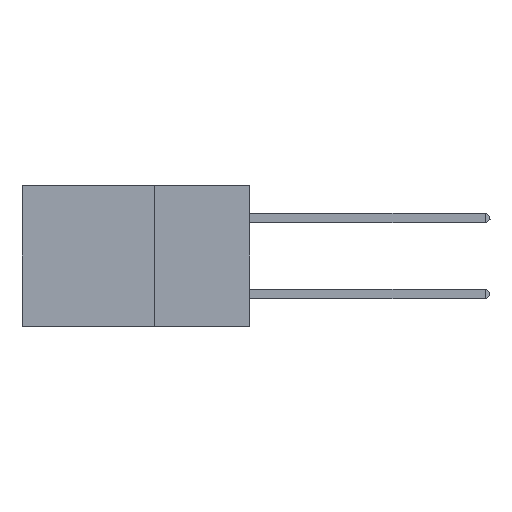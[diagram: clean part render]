
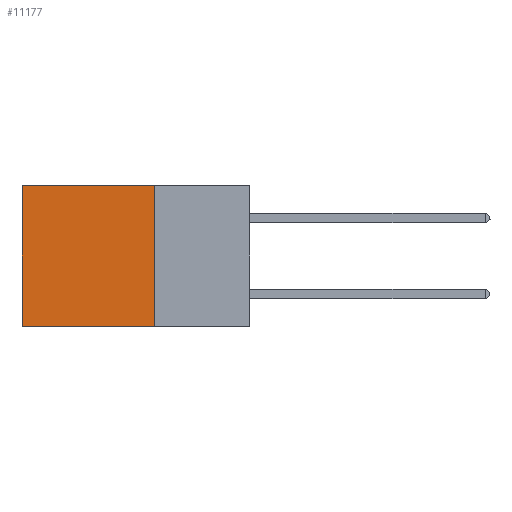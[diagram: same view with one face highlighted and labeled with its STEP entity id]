
A CAD part, left-side view. The second image highlights one B-rep face of the part: STEP entity #11177.
In plain terms, the highlighted planar face has unit normal (-1, 0, 0).
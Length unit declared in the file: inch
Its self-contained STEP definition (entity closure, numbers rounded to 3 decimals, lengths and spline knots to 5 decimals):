
#91 = CARTESIAN_POINT ( 'NONE',  ( 0.2875, 0.25, -0.37 ) ) ;
#647 = EDGE_CURVE ( 'NONE', #10352, #7145, #11115, .T. ) ;
#807 = LINE ( 'NONE', #5110, #1570 ) ;
#1309 = VERTEX_POINT ( 'NONE', #1492 ) ;
#1450 = VECTOR ( 'NONE', #3809, 39.37008 ) ;
#1492 = CARTESIAN_POINT ( 'NONE',  ( 0.2875, 0.25, 0. ) ) ;
#1570 = VECTOR ( 'NONE', #4062, 39.37008 ) ;
#2168 = AXIS2_PLACEMENT_3D ( 'NONE', #12699, #11774, #2237 ) ;
#2237 = DIRECTION ( 'NONE',  ( 0., 0., -1. ) ) ;
#2741 = LINE ( 'NONE', #13353, #1450 ) ;
#3264 = VECTOR ( 'NONE', #4398, 39.37008 ) ;
#3532 = CARTESIAN_POINT ( 'NONE',  ( 0.2875, 0.25, -0.37 ) ) ;
#3626 = ORIENTED_EDGE ( 'NONE', *, *, #4147, .F. ) ;
#3809 = DIRECTION ( 'NONE',  ( 0., 1., 0. ) ) ;
#4062 = DIRECTION ( 'NONE',  ( 0., 0., -1. ) ) ;
#4147 = EDGE_CURVE ( 'NONE', #1309, #10352, #807, .T. ) ;
#4398 = DIRECTION ( 'NONE',  ( 0., 1., 0. ) ) ;
#5110 = CARTESIAN_POINT ( 'NONE',  ( 0.2875, 0.25, 0. ) ) ;
#5256 = ORIENTED_EDGE ( 'NONE', *, *, #10356, .T. ) ;
#5504 = VECTOR ( 'NONE', #7797, 39.37008 ) ;
#6137 = CARTESIAN_POINT ( 'NONE',  ( 0.2875, 0.6, 0. ) ) ;
#6767 = VERTEX_POINT ( 'NONE', #6137 ) ;
#6969 = CARTESIAN_POINT ( 'NONE',  ( 0.2875, 0.6, -0.37 ) ) ;
#7145 = VERTEX_POINT ( 'NONE', #6969 ) ;
#7778 = EDGE_LOOP ( 'NONE', ( #5256, #10791, #3626, #10178 ) ) ;
#7797 = DIRECTION ( 'NONE',  ( 0., 0., -1. ) ) ;
#9211 = EDGE_CURVE ( 'NONE', #1309, #6767, #2741, .T. ) ;
#10178 = ORIENTED_EDGE ( 'NONE', *, *, #9211, .T. ) ;
#10352 = VERTEX_POINT ( 'NONE', #3532 ) ;
#10356 = EDGE_CURVE ( 'NONE', #6767, #7145, #12929, .T. ) ;
#10665 = PLANE ( 'NONE',  #2168 ) ;
#10791 = ORIENTED_EDGE ( 'NONE', *, *, #647, .F. ) ;
#11115 = LINE ( 'NONE', #91, #3264 ) ;
#11177 = ADVANCED_FACE ( 'NONE', ( #11846 ), #10665, .F. ) ;
#11774 = DIRECTION ( 'NONE',  ( 1., 0., 0. ) ) ;
#11846 = FACE_OUTER_BOUND ( 'NONE', #7778, .T. ) ;
#12699 = CARTESIAN_POINT ( 'NONE',  ( 0.2875, 0.25, 0. ) ) ;
#12929 = LINE ( 'NONE', #13222, #5504 ) ;
#13222 = CARTESIAN_POINT ( 'NONE',  ( 0.2875, 0.6, 0. ) ) ;
#13353 = CARTESIAN_POINT ( 'NONE',  ( 0.2875, 0.25, 0. ) ) ;
